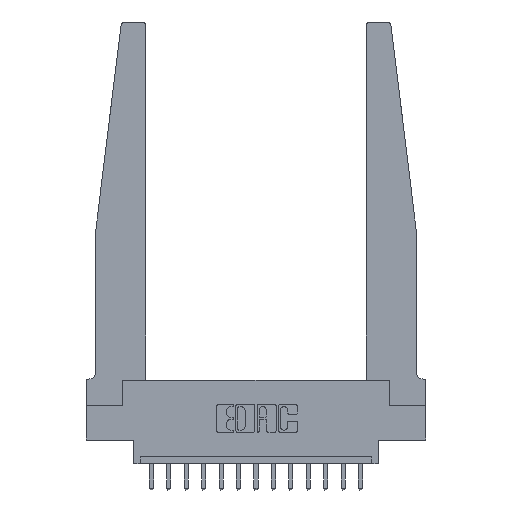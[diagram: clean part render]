
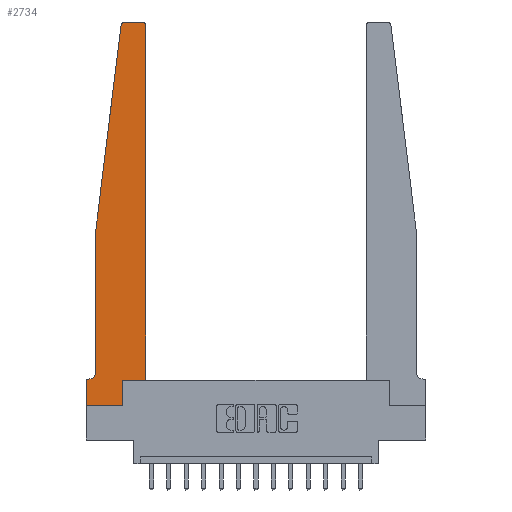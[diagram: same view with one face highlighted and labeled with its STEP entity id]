
A CAD part, top view. The second image highlights one B-rep face of the part: STEP entity #2734.
In plain terms, the highlighted planar face has unit normal (0, 0, 1).
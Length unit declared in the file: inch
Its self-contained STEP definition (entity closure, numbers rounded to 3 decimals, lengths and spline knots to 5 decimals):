
#11 = DIRECTION ( 'NONE',  ( 0., 0., 1. ) ) ;
#256 = LINE ( 'NONE', #14046, #6420 ) ;
#522 = CARTESIAN_POINT ( 'NONE',  ( 0.425, 0.18, 0.37 ) ) ;
#577 = DIRECTION ( 'NONE',  ( 0., 0., 1. ) ) ;
#640 = LINE ( 'NONE', #8690, #1857 ) ;
#947 = CARTESIAN_POINT ( 'NONE',  ( 0.065, 0.2375, 0.37 ) ) ;
#1157 = EDGE_CURVE ( 'NONE', #4807, #8002, #256, .T. ) ;
#1233 = AXIS2_PLACEMENT_3D ( 'NONE', #14958, #577, #5625 ) ;
#1420 = VERTEX_POINT ( 'NONE', #5449 ) ;
#1557 = DIRECTION ( 'NONE',  ( 1., 0., 0. ) ) ;
#1722 = CARTESIAN_POINT ( 'NONE',  ( 0., 0.1875, 0.37 ) ) ;
#1857 = VECTOR ( 'NONE', #9119, 39.37008 ) ;
#1904 = LINE ( 'NONE', #5240, #10376 ) ;
#1943 = VERTEX_POINT ( 'NONE', #12038 ) ;
#2069 = EDGE_CURVE ( 'NONE', #14782, #4807, #640, .T. ) ;
#2142 = DIRECTION ( 'NONE',  ( 0., -1., 0. ) ) ;
#2163 = FACE_OUTER_BOUND ( 'NONE', #4390, .T. ) ;
#2421 = ORIENTED_EDGE ( 'NONE', *, *, #14159, .T. ) ;
#2498 = CARTESIAN_POINT ( 'NONE',  ( 0.065, 1.25, 0.37 ) ) ;
#2525 = VECTOR ( 'NONE', #11496, 39.37008 ) ;
#2728 = VERTEX_POINT ( 'NONE', #7584 ) ;
#2734 = ADVANCED_FACE ( 'NONE', ( #2163 ), #11491, .T. ) ;
#2857 = EDGE_CURVE ( 'NONE', #1420, #1943, #8143, .T. ) ;
#2872 = ORIENTED_EDGE ( 'NONE', *, *, #3809, .T. ) ;
#2974 = VECTOR ( 'NONE', #7007, 39.37008 ) ;
#3741 = VECTOR ( 'NONE', #1557, 39.37008 ) ;
#3809 = EDGE_CURVE ( 'NONE', #10074, #9483, #1904, .T. ) ;
#4022 = VERTEX_POINT ( 'NONE', #947 ) ;
#4204 = CIRCLE ( 'NONE', #13631, 0.03 ) ;
#4236 = EDGE_CURVE ( 'NONE', #7058, #10074, #6007, .T. ) ;
#4390 = EDGE_LOOP ( 'NONE', ( #4555, #6525, #12697, #13465, #5190, #13600, #6028, #12857, #2421, #14814, #2872, #6668 ) ) ;
#4460 = CIRCLE ( 'NONE', #9212, 0.05 ) ;
#4555 = ORIENTED_EDGE ( 'NONE', *, *, #11324, .T. ) ;
#4664 = DIRECTION ( 'NONE',  ( -1., 0., 0. ) ) ;
#4751 = CARTESIAN_POINT ( 'NONE',  ( 0.27653, 2.72, 0.37 ) ) ;
#4806 = DIRECTION ( 'NONE',  ( 1., 0., 0. ) ) ;
#4807 = VERTEX_POINT ( 'NONE', #1722 ) ;
#4866 = EDGE_CURVE ( 'NONE', #9483, #11207, #7216, .T. ) ;
#5190 = ORIENTED_EDGE ( 'NONE', *, *, #8201, .T. ) ;
#5240 = CARTESIAN_POINT ( 'NONE',  ( 0.425, 0.18, 0.37 ) ) ;
#5449 = CARTESIAN_POINT ( 'NONE',  ( 0.24675, 2.72367, 0.37 ) ) ;
#5625 = DIRECTION ( 'NONE',  ( 1., 0., 0. ) ) ;
#5820 = CARTESIAN_POINT ( 'NONE',  ( 0.425, 2.72, 0.37 ) ) ;
#5847 = AXIS2_PLACEMENT_3D ( 'NONE', #8976, #7990, #10525 ) ;
#6005 = VECTOR ( 'NONE', #15489, 39.37008 ) ;
#6007 = LINE ( 'NONE', #6084, #2525 ) ;
#6028 = ORIENTED_EDGE ( 'NONE', *, *, #1157, .T. ) ;
#6084 = CARTESIAN_POINT ( 'NONE',  ( 0.425, 0.18, 0.37 ) ) ;
#6420 = VECTOR ( 'NONE', #2142, 39.37008 ) ;
#6525 = ORIENTED_EDGE ( 'NONE', *, *, #10201, .T. ) ;
#6668 = ORIENTED_EDGE ( 'NONE', *, *, #4866, .T. ) ;
#6879 = CARTESIAN_POINT ( 'NONE',  ( 0.2605, 0.18, 0.37 ) ) ;
#7007 = DIRECTION ( 'NONE',  ( -0.122, -0.992, 0. ) ) ;
#7058 = VERTEX_POINT ( 'NONE', #12858 ) ;
#7216 = CIRCLE ( 'NONE', #1233, 0.03 ) ;
#7225 = CARTESIAN_POINT ( 'NONE',  ( 0.065, 1.25, 0.37 ) ) ;
#7230 = LINE ( 'NONE', #9457, #3741 ) ;
#7584 = CARTESIAN_POINT ( 'NONE',  ( 0.27653, 2.75, 0.37 ) ) ;
#7771 = CARTESIAN_POINT ( 'NONE',  ( 0., 0., 0.37 ) ) ;
#7870 = LINE ( 'NONE', #2498, #6005 ) ;
#7990 = DIRECTION ( 'NONE',  ( 0., 0., 1. ) ) ;
#8002 = VERTEX_POINT ( 'NONE', #7771 ) ;
#8143 = LINE ( 'NONE', #7225, #2974 ) ;
#8201 = EDGE_CURVE ( 'NONE', #4022, #14782, #4460, .T. ) ;
#8287 = CARTESIAN_POINT ( 'NONE',  ( 0.015, 0.1875, 0.37 ) ) ;
#8690 = CARTESIAN_POINT ( 'NONE',  ( 0.065, 0.1875, 0.37 ) ) ;
#8976 = CARTESIAN_POINT ( 'NONE',  ( 0., 0.1875, 0.37 ) ) ;
#9119 = DIRECTION ( 'NONE',  ( -1., 0., 0. ) ) ;
#9212 = AXIS2_PLACEMENT_3D ( 'NONE', #13977, #13789, #4664 ) ;
#9234 = DIRECTION ( 'NONE',  ( 0., 1., 0. ) ) ;
#9457 = CARTESIAN_POINT ( 'NONE',  ( 0., 0., 0.37 ) ) ;
#9483 = VERTEX_POINT ( 'NONE', #5820 ) ;
#10074 = VERTEX_POINT ( 'NONE', #522 ) ;
#10201 = EDGE_CURVE ( 'NONE', #2728, #1420, #4204, .T. ) ;
#10376 = VECTOR ( 'NONE', #9234, 39.37008 ) ;
#10525 = DIRECTION ( 'NONE',  ( 1., 0., 0. ) ) ;
#10976 = DIRECTION ( 'NONE',  ( 0., 1., 0. ) ) ;
#11162 = EDGE_CURVE ( 'NONE', #1943, #4022, #7870, .T. ) ;
#11207 = VERTEX_POINT ( 'NONE', #12897 ) ;
#11324 = EDGE_CURVE ( 'NONE', #11207, #2728, #13825, .T. ) ;
#11477 = EDGE_CURVE ( 'NONE', #8002, #14379, #7230, .T. ) ;
#11491 = PLANE ( 'NONE',  #5847 ) ;
#11496 = DIRECTION ( 'NONE',  ( 1., 0., 0. ) ) ;
#11921 = CARTESIAN_POINT ( 'NONE',  ( 0.25, 2.75, 0.37 ) ) ;
#12038 = CARTESIAN_POINT ( 'NONE',  ( 0.065, 1.25, 0.37 ) ) ;
#12697 = ORIENTED_EDGE ( 'NONE', *, *, #2857, .T. ) ;
#12857 = ORIENTED_EDGE ( 'NONE', *, *, #11477, .T. ) ;
#12858 = CARTESIAN_POINT ( 'NONE',  ( 0.2605, 0.18, 0.37 ) ) ;
#12897 = CARTESIAN_POINT ( 'NONE',  ( 0.395, 2.75, 0.37 ) ) ;
#13014 = DIRECTION ( 'NONE',  ( -1., 0., 0. ) ) ;
#13465 = ORIENTED_EDGE ( 'NONE', *, *, #11162, .T. ) ;
#13537 = VECTOR ( 'NONE', #10976, 39.37008 ) ;
#13600 = ORIENTED_EDGE ( 'NONE', *, *, #2069, .T. ) ;
#13631 = AXIS2_PLACEMENT_3D ( 'NONE', #4751, #11, #4806 ) ;
#13789 = DIRECTION ( 'NONE',  ( 0., 0., -1. ) ) ;
#13825 = LINE ( 'NONE', #11921, #15658 ) ;
#13977 = CARTESIAN_POINT ( 'NONE',  ( 0.015, 0.2375, 0.37 ) ) ;
#13990 = CARTESIAN_POINT ( 'NONE',  ( 0.2605, 0., 0.37 ) ) ;
#14046 = CARTESIAN_POINT ( 'NONE',  ( 0., 0., 0.37 ) ) ;
#14159 = EDGE_CURVE ( 'NONE', #14379, #7058, #14380, .T. ) ;
#14379 = VERTEX_POINT ( 'NONE', #13990 ) ;
#14380 = LINE ( 'NONE', #6879, #13537 ) ;
#14782 = VERTEX_POINT ( 'NONE', #8287 ) ;
#14814 = ORIENTED_EDGE ( 'NONE', *, *, #4236, .T. ) ;
#14958 = CARTESIAN_POINT ( 'NONE',  ( 0.395, 2.72, 0.37 ) ) ;
#15489 = DIRECTION ( 'NONE',  ( 0., -1., 0. ) ) ;
#15658 = VECTOR ( 'NONE', #13014, 39.37008 ) ;
